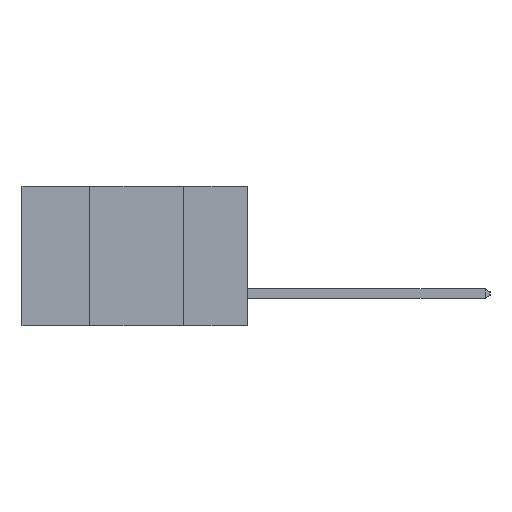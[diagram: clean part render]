
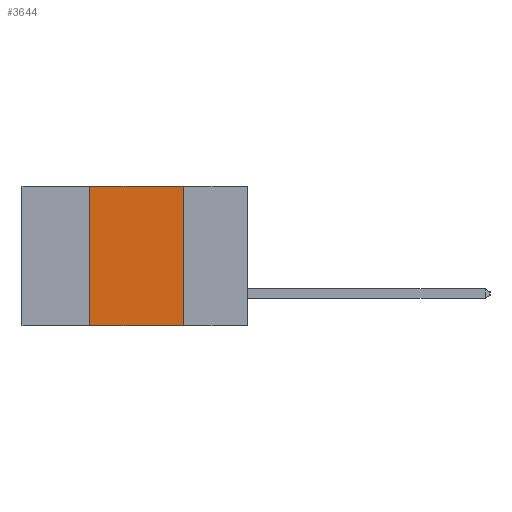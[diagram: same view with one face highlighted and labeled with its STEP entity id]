
A CAD part, left-side view. The second image highlights one B-rep face of the part: STEP entity #3644.
In plain terms, the highlighted planar face has unit normal (-1, 0, 0).
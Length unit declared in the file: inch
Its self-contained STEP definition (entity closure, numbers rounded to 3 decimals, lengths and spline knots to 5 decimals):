
#462 = CARTESIAN_POINT ( 'NONE',  ( 0., 0.17, -0.37 ) ) ;
#479 = CARTESIAN_POINT ( 'NONE',  ( 0., 0.17, -0.37 ) ) ;
#1728 = CARTESIAN_POINT ( 'NONE',  ( 0., 0.6, 0. ) ) ;
#1817 = VERTEX_POINT ( 'NONE', #462 ) ;
#2502 = LINE ( 'NONE', #1728, #18080 ) ;
#3644 = ADVANCED_FACE ( 'NONE', ( #16951 ), #15310, .F. ) ;
#3744 = ORIENTED_EDGE ( 'NONE', *, *, #17825, .F. ) ;
#4004 = EDGE_CURVE ( 'NONE', #10414, #1817, #7434, .T. ) ;
#5991 = ORIENTED_EDGE ( 'NONE', *, *, #4004, .T. ) ;
#7434 = LINE ( 'NONE', #10157, #12193 ) ;
#7458 = VECTOR ( 'NONE', #22041, 39.37008 ) ;
#7672 = CARTESIAN_POINT ( 'NONE',  ( 0., 0.42, 0. ) ) ;
#8815 = DIRECTION ( 'NONE',  ( 0., 0., -1. ) ) ;
#9925 = DIRECTION ( 'NONE',  ( 0., -1., 0. ) ) ;
#10157 = CARTESIAN_POINT ( 'NONE',  ( 0., 0.6, -0.37 ) ) ;
#10414 = VERTEX_POINT ( 'NONE', #17651 ) ;
#12193 = VECTOR ( 'NONE', #9925, 39.37008 ) ;
#12653 = LINE ( 'NONE', #479, #22665 ) ;
#13369 = VERTEX_POINT ( 'NONE', #20618 ) ;
#13997 = DIRECTION ( 'NONE',  ( 0., -1., 0. ) ) ;
#14017 = CARTESIAN_POINT ( 'NONE',  ( 0., 0.42, -0.37 ) ) ;
#14476 = EDGE_CURVE ( 'NONE', #16260, #13369, #2502, .T. ) ;
#15230 = DIRECTION ( 'NONE',  ( 0., 0., -1. ) ) ;
#15279 = DIRECTION ( 'NONE',  ( 1., 0., 0. ) ) ;
#15310 = PLANE ( 'NONE',  #18333 ) ;
#15543 = CARTESIAN_POINT ( 'NONE',  ( 0., 0.6, 0. ) ) ;
#16260 = VERTEX_POINT ( 'NONE', #7672 ) ;
#16951 = FACE_OUTER_BOUND ( 'NONE', #25190, .T. ) ;
#17651 = CARTESIAN_POINT ( 'NONE',  ( 0., 0.42, -0.37 ) ) ;
#17825 = EDGE_CURVE ( 'NONE', #13369, #1817, #12653, .T. ) ;
#18080 = VECTOR ( 'NONE', #13997, 39.37008 ) ;
#18333 = AXIS2_PLACEMENT_3D ( 'NONE', #15543, #15279, #15230 ) ;
#18659 = ORIENTED_EDGE ( 'NONE', *, *, #20916, .F. ) ;
#20618 = CARTESIAN_POINT ( 'NONE',  ( 0., 0.17, 0. ) ) ;
#20916 = EDGE_CURVE ( 'NONE', #10414, #16260, #23476, .T. ) ;
#22041 = DIRECTION ( 'NONE',  ( 0., 0., 1. ) ) ;
#22665 = VECTOR ( 'NONE', #8815, 39.37008 ) ;
#23476 = LINE ( 'NONE', #14017, #7458 ) ;
#24585 = ORIENTED_EDGE ( 'NONE', *, *, #14476, .F. ) ;
#25190 = EDGE_LOOP ( 'NONE', ( #3744, #24585, #18659, #5991 ) ) ;
